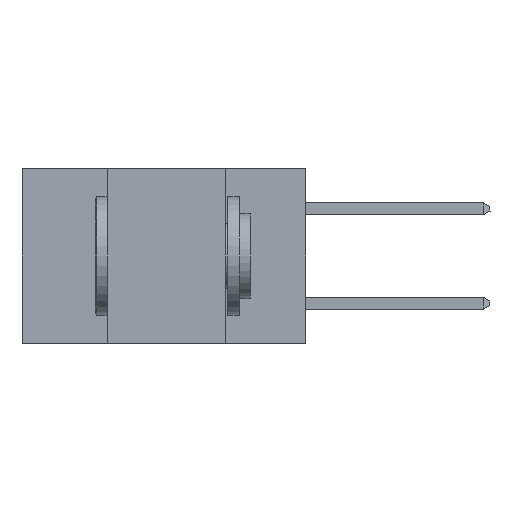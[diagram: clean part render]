
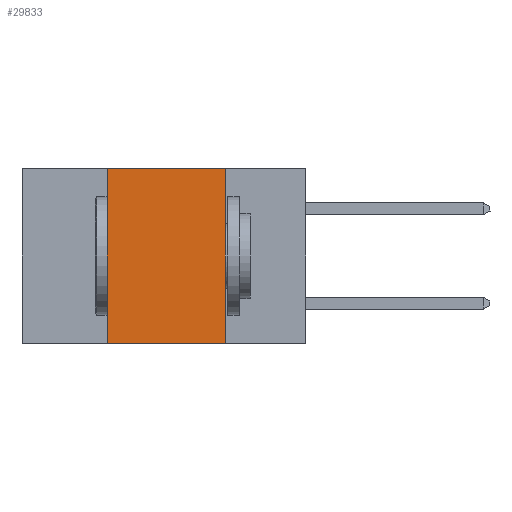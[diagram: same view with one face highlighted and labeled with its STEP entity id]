
A CAD part, left-side view. The second image highlights one B-rep face of the part: STEP entity #29833.
In plain terms, the highlighted planar face has unit normal (-1, 0, 0).
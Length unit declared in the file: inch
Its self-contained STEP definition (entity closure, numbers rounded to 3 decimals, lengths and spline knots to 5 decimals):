
#1687 = ORIENTED_EDGE ( 'NONE', *, *, #25829, .T. ) ;
#2103 = FACE_OUTER_BOUND ( 'NONE', #8872, .T. ) ;
#2355 = CARTESIAN_POINT ( 'NONE',  ( 0., 0.6, 0. ) ) ;
#2615 = AXIS2_PLACEMENT_3D ( 'NONE', #6752, #18795, #14187 ) ;
#3900 = EDGE_CURVE ( 'NONE', #17821, #14477, #9730, .T. ) ;
#4694 = VECTOR ( 'NONE', #11299, 39.37008 ) ;
#6752 = CARTESIAN_POINT ( 'NONE',  ( 0., 0.6, 0. ) ) ;
#8872 = EDGE_LOOP ( 'NONE', ( #20735, #29842, #18325, #1687 ) ) ;
#9730 = LINE ( 'NONE', #2355, #22067 ) ;
#11299 = DIRECTION ( 'NONE',  ( 0., 0., -1. ) ) ;
#12121 = CARTESIAN_POINT ( 'NONE',  ( 0., 0.42, -0.37 ) ) ;
#13932 = DIRECTION ( 'NONE',  ( 0., 0., 1. ) ) ;
#14187 = DIRECTION ( 'NONE',  ( 0., 0., -1. ) ) ;
#14477 = VERTEX_POINT ( 'NONE', #24160 ) ;
#15646 = CARTESIAN_POINT ( 'NONE',  ( 0., 0.42, 0. ) ) ;
#16807 = DIRECTION ( 'NONE',  ( 0., -1., 0. ) ) ;
#17821 = VERTEX_POINT ( 'NONE', #15646 ) ;
#18325 = ORIENTED_EDGE ( 'NONE', *, *, #27785, .F. ) ;
#18795 = DIRECTION ( 'NONE',  ( 1., 0., 0. ) ) ;
#19374 = VECTOR ( 'NONE', #13932, 39.37008 ) ;
#20735 = ORIENTED_EDGE ( 'NONE', *, *, #29594, .F. ) ;
#20812 = VERTEX_POINT ( 'NONE', #12121 ) ;
#21211 = DIRECTION ( 'NONE',  ( 0., -1., 0. ) ) ;
#21246 = LINE ( 'NONE', #23814, #26038 ) ;
#22067 = VECTOR ( 'NONE', #16807, 39.37008 ) ;
#23011 = CARTESIAN_POINT ( 'NONE',  ( 0., 0.17, 0. ) ) ;
#23751 = LINE ( 'NONE', #23011, #4694 ) ;
#23814 = CARTESIAN_POINT ( 'NONE',  ( 0., 0.6, -0.37 ) ) ;
#24160 = CARTESIAN_POINT ( 'NONE',  ( 0., 0.17, 0. ) ) ;
#24189 = LINE ( 'NONE', #30532, #19374 ) ;
#25829 = EDGE_CURVE ( 'NONE', #20812, #29990, #21246, .T. ) ;
#26038 = VECTOR ( 'NONE', #21211, 39.37008 ) ;
#27785 = EDGE_CURVE ( 'NONE', #20812, #17821, #24189, .T. ) ;
#28195 = PLANE ( 'NONE',  #2615 ) ;
#29302 = CARTESIAN_POINT ( 'NONE',  ( 0., 0.17, -0.37 ) ) ;
#29594 = EDGE_CURVE ( 'NONE', #14477, #29990, #23751, .T. ) ;
#29833 = ADVANCED_FACE ( 'NONE', ( #2103 ), #28195, .F. ) ;
#29842 = ORIENTED_EDGE ( 'NONE', *, *, #3900, .F. ) ;
#29990 = VERTEX_POINT ( 'NONE', #29302 ) ;
#30532 = CARTESIAN_POINT ( 'NONE',  ( 0., 0.42, 0. ) ) ;
